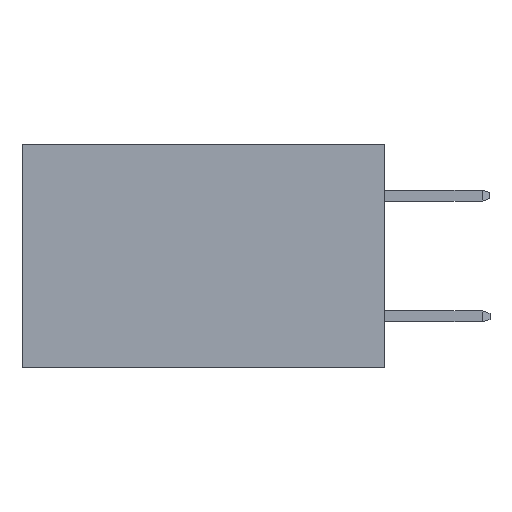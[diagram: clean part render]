
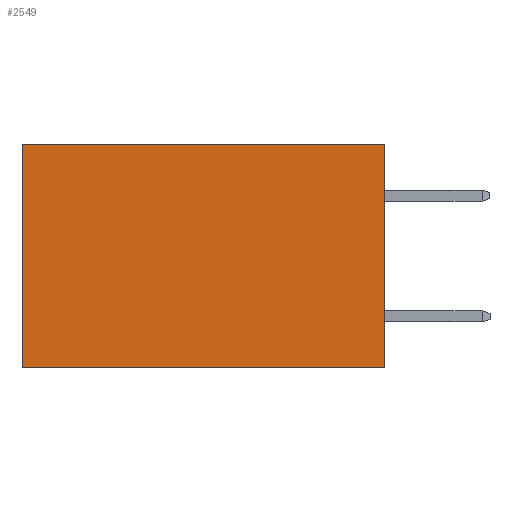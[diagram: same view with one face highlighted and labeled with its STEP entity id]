
A CAD part, left-side view. The second image highlights one B-rep face of the part: STEP entity #2549.
In plain terms, the highlighted planar face has unit normal (-1, 0, 0).
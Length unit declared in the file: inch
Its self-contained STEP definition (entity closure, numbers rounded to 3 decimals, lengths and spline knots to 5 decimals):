
#114 = ORIENTED_EDGE ( 'NONE', *, *, #5650, .T. ) ;
#513 = CARTESIAN_POINT ( 'NONE',  ( 0.2615, 0., 0. ) ) ;
#738 = VERTEX_POINT ( 'NONE', #3953 ) ;
#1031 = VERTEX_POINT ( 'NONE', #6509 ) ;
#1548 = ORIENTED_EDGE ( 'NONE', *, *, #3286, .F. ) ;
#1859 = CARTESIAN_POINT ( 'NONE',  ( 0.2615, 0., -0.37 ) ) ;
#2549 = ADVANCED_FACE ( 'NONE', ( #3214 ), #5383, .F. ) ;
#2653 = EDGE_CURVE ( 'NONE', #5437, #1031, #8028, .T. ) ;
#3214 = FACE_OUTER_BOUND ( 'NONE', #6016, .T. ) ;
#3248 = VECTOR ( 'NONE', #6356, 39.37008 ) ;
#3286 = EDGE_CURVE ( 'NONE', #7214, #738, #3367, .T. ) ;
#3367 = LINE ( 'NONE', #7120, #6287 ) ;
#3495 = AXIS2_PLACEMENT_3D ( 'NONE', #4998, #4972, #6290 ) ;
#3543 = EDGE_CURVE ( 'NONE', #5437, #7214, #7153, .T. ) ;
#3881 = ORIENTED_EDGE ( 'NONE', *, *, #2653, .T. ) ;
#3953 = CARTESIAN_POINT ( 'NONE',  ( 0.2615, 0.6, -0.37 ) ) ;
#4812 = VECTOR ( 'NONE', #6606, 39.37008 ) ;
#4972 = DIRECTION ( 'NONE',  ( 1., 0., 0. ) ) ;
#4998 = CARTESIAN_POINT ( 'NONE',  ( 0.2615, 0., -0.37 ) ) ;
#5383 = PLANE ( 'NONE',  #3495 ) ;
#5437 = VERTEX_POINT ( 'NONE', #513 ) ;
#5529 = VECTOR ( 'NONE', #7482, 39.37008 ) ;
#5650 = EDGE_CURVE ( 'NONE', #1031, #738, #8162, .T. ) ;
#6016 = EDGE_LOOP ( 'NONE', ( #114, #1548, #7596, #3881 ) ) ;
#6287 = VECTOR ( 'NONE', #7069, 39.37008 ) ;
#6290 = DIRECTION ( 'NONE',  ( 0., 0., -1. ) ) ;
#6356 = DIRECTION ( 'NONE',  ( 0., 0., -1. ) ) ;
#6509 = CARTESIAN_POINT ( 'NONE',  ( 0.2615, 0.6, 0. ) ) ;
#6606 = DIRECTION ( 'NONE',  ( 0., 1., 0. ) ) ;
#6635 = CARTESIAN_POINT ( 'NONE',  ( 0.2615, 0., -0.37 ) ) ;
#6733 = CARTESIAN_POINT ( 'NONE',  ( 0.2615, 0., 0. ) ) ;
#6912 = CARTESIAN_POINT ( 'NONE',  ( 0.2615, 0.6, -0.37 ) ) ;
#7069 = DIRECTION ( 'NONE',  ( 0., 1., 0. ) ) ;
#7120 = CARTESIAN_POINT ( 'NONE',  ( 0.2615, 0., -0.37 ) ) ;
#7153 = LINE ( 'NONE', #6635, #5529 ) ;
#7214 = VERTEX_POINT ( 'NONE', #1859 ) ;
#7482 = DIRECTION ( 'NONE',  ( 0., 0., -1. ) ) ;
#7596 = ORIENTED_EDGE ( 'NONE', *, *, #3543, .F. ) ;
#8028 = LINE ( 'NONE', #6733, #4812 ) ;
#8162 = LINE ( 'NONE', #6912, #3248 ) ;
